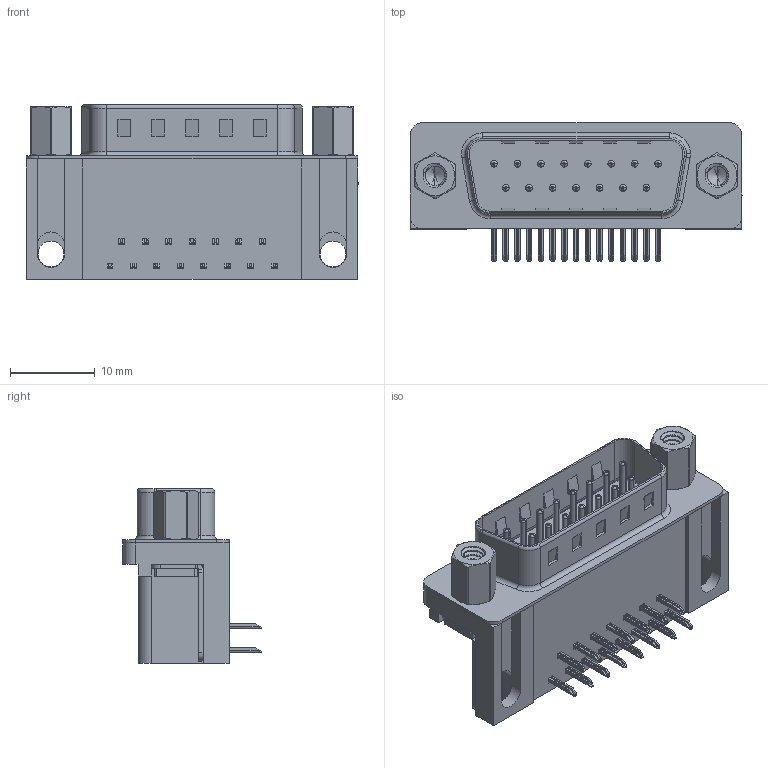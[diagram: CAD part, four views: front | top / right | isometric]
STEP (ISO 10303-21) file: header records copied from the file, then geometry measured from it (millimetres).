
FILE_DESCRIPTION (( 'STEP AP203' ), '1' );
FILE_NAME ('629-015-340-513.STEP', '2021-09-21T20:15:48', ( '' ), ( '' ), 'SwSTEP 2.0', 'SolidWorks 2020', '' );
FILE_SCHEMA (( 'CONFIG_CONTROL_DESIGN' ));
Length unit declared in the file: millimetre
Products named in the file (8): 629 4-40 Threaded Rivet; 629 Contact Bottom; 629 4-40 Hex Standoff 5; 629 Housing_15 Socket; 629 Thru Hole Board Mount; 629 Shell_15 Socket; 629-015-340-513; 629 Contact Top
Assembly tree (23 placements, depth 2):
  629-015-340-513
    629 Housing_15 Socket
    629 Shell_15 Socket
    629 Contact Bottom  x7
    629 Contact Top  x8
    629 Thru Hole Board Mount  x2
    629 4-40 Threaded Rivet  x2
    629 4-40 Hex Standoff 5  x2
Bounding box: 39.22 x 16.35 x 20.6 mm (x, y, z)
Volume: 5288.8 mm3; surface area: 6523.9 mm2
Topology: 23 solids, 23 shells, 1601 faces, 4021 edges, 2503 vertices
Faces by surface type: plane 913, cylinder 517, torus 121, cone 32, bspline 18
Entity records: 23660 total; most frequent: CARTESIAN_POINT 7807, ORIENTED_EDGE 3042, DIRECTION 3035, EDGE_CURVE 1521, AXIS2_PLACEMENT_3D 1033, VERTEX_POINT 974, VECTOR 969, LINE 969
